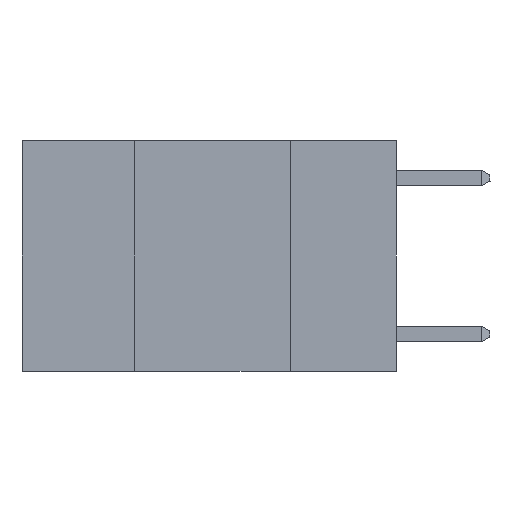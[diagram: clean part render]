
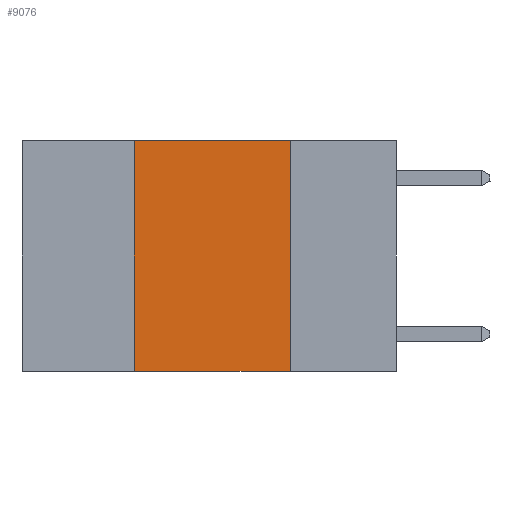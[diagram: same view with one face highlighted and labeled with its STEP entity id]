
A CAD part, left-side view. The second image highlights one B-rep face of the part: STEP entity #9076.
In plain terms, the highlighted planar face has unit normal (-1, 0, 0).
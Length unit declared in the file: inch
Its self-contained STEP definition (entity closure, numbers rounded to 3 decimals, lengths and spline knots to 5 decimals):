
#44 = EDGE_CURVE ( 'NONE', #2300, #8379, #6302, .T. ) ;
#902 = CARTESIAN_POINT ( 'NONE',  ( 0., 0.42, -0.37 ) ) ;
#1492 = VECTOR ( 'NONE', #1986, 39.37008 ) ;
#1647 = EDGE_CURVE ( 'NONE', #8379, #4403, #8207, .T. ) ;
#1812 = FACE_OUTER_BOUND ( 'NONE', #5597, .T. ) ;
#1986 = DIRECTION ( 'NONE',  ( 0., -1., 0. ) ) ;
#2104 = ORIENTED_EDGE ( 'NONE', *, *, #44, .F. ) ;
#2300 = VERTEX_POINT ( 'NONE', #6046 ) ;
#2374 = PLANE ( 'NONE',  #6318 ) ;
#2724 = CARTESIAN_POINT ( 'NONE',  ( 0., 0.17, 0. ) ) ;
#2906 = CARTESIAN_POINT ( 'NONE',  ( 0., 0.6, 0. ) ) ;
#3243 = DIRECTION ( 'NONE',  ( 0., 0., -1. ) ) ;
#3931 = VECTOR ( 'NONE', #4102, 39.37008 ) ;
#3961 = CARTESIAN_POINT ( 'NONE',  ( 0., 0.42, 0. ) ) ;
#4102 = DIRECTION ( 'NONE',  ( 0., 0., -1. ) ) ;
#4403 = VERTEX_POINT ( 'NONE', #6440 ) ;
#4891 = CARTESIAN_POINT ( 'NONE',  ( 0., 0.6, 0. ) ) ;
#5047 = EDGE_CURVE ( 'NONE', #5601, #2300, #9744, .T. ) ;
#5597 = EDGE_LOOP ( 'NONE', ( #10326, #2104, #8584, #8823 ) ) ;
#5601 = VERTEX_POINT ( 'NONE', #902 ) ;
#5621 = CARTESIAN_POINT ( 'NONE',  ( 0., 0.17, 0. ) ) ;
#6031 = VECTOR ( 'NONE', #7583, 39.37008 ) ;
#6046 = CARTESIAN_POINT ( 'NONE',  ( 0., 0.42, 0. ) ) ;
#6302 = LINE ( 'NONE', #2906, #6031 ) ;
#6318 = AXIS2_PLACEMENT_3D ( 'NONE', #4891, #8080, #3243 ) ;
#6440 = CARTESIAN_POINT ( 'NONE',  ( 0., 0.17, -0.37 ) ) ;
#7263 = VECTOR ( 'NONE', #10208, 39.37008 ) ;
#7583 = DIRECTION ( 'NONE',  ( 0., -1., 0. ) ) ;
#7720 = EDGE_CURVE ( 'NONE', #5601, #4403, #7808, .T. ) ;
#7808 = LINE ( 'NONE', #9970, #1492 ) ;
#8080 = DIRECTION ( 'NONE',  ( 1., 0., 0. ) ) ;
#8207 = LINE ( 'NONE', #2724, #3931 ) ;
#8379 = VERTEX_POINT ( 'NONE', #5621 ) ;
#8584 = ORIENTED_EDGE ( 'NONE', *, *, #5047, .F. ) ;
#8823 = ORIENTED_EDGE ( 'NONE', *, *, #7720, .T. ) ;
#9076 = ADVANCED_FACE ( 'NONE', ( #1812 ), #2374, .F. ) ;
#9744 = LINE ( 'NONE', #3961, #7263 ) ;
#9970 = CARTESIAN_POINT ( 'NONE',  ( 0., 0.6, -0.37 ) ) ;
#10208 = DIRECTION ( 'NONE',  ( 0., 0., 1. ) ) ;
#10326 = ORIENTED_EDGE ( 'NONE', *, *, #1647, .F. ) ;
